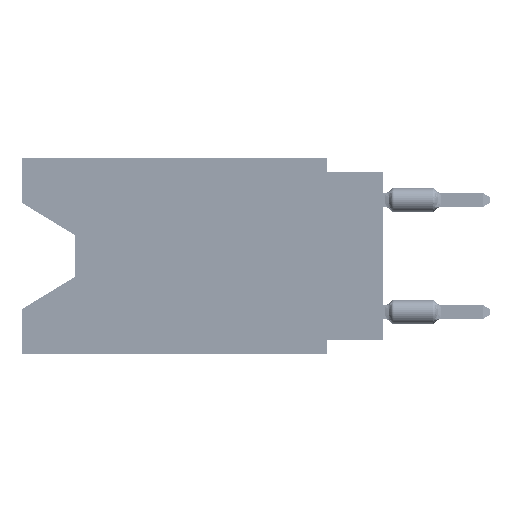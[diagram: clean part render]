
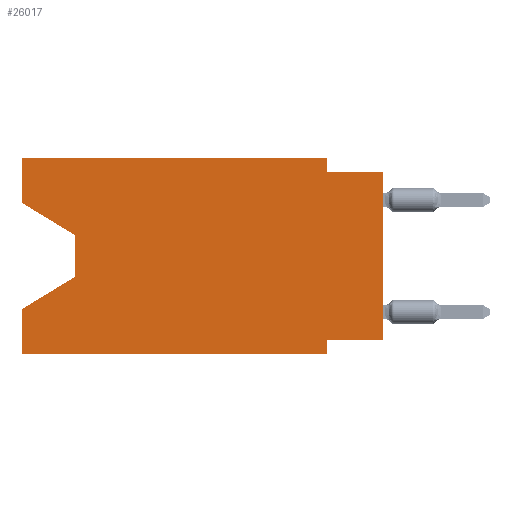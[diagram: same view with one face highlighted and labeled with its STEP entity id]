
A CAD part, left-side view. The second image highlights one B-rep face of the part: STEP entity #26017.
In plain terms, the highlighted planar face has unit normal (-1, 0, 0).
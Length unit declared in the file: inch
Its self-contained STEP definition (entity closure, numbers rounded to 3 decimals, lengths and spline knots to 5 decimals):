
#196 = DIRECTION ( 'NONE',  ( 0., 0., 1. ) ) ;
#645 = LINE ( 'NONE', #35920, #61650 ) ;
#1305 = EDGE_CURVE ( 'NONE', #66313, #22376, #6576, .T. ) ;
#3729 = FACE_OUTER_BOUND ( 'NONE', #34049, .T. ) ;
#4725 = CARTESIAN_POINT ( 'NONE',  ( 0., 0.1, -0.325 ) ) ;
#5336 = VECTOR ( 'NONE', #64543, 39.37008 ) ;
#5364 = VECTOR ( 'NONE', #60416, 39.37008 ) ;
#6576 = LINE ( 'NONE', #7235, #58800 ) ;
#7235 = CARTESIAN_POINT ( 'NONE',  ( 0., 0., 0. ) ) ;
#7884 = VECTOR ( 'NONE', #54896, 39.37008 ) ;
#8128 = LINE ( 'NONE', #8451, #54792 ) ;
#8451 = CARTESIAN_POINT ( 'NONE',  ( 0., 0.1, 0. ) ) ;
#8800 = VERTEX_POINT ( 'NONE', #4725 ) ;
#9898 = CARTESIAN_POINT ( 'NONE',  ( 0., 0.1, -0.025 ) ) ;
#12039 = CARTESIAN_POINT ( 'NONE',  ( 0., 0.55, -0.212 ) ) ;
#14314 = ORIENTED_EDGE ( 'NONE', *, *, #38287, .T. ) ;
#14531 = VERTEX_POINT ( 'NONE', #9898 ) ;
#15044 = LINE ( 'NONE', #24134, #5364 ) ;
#15332 = ORIENTED_EDGE ( 'NONE', *, *, #54161, .F. ) ;
#15468 = DIRECTION ( 'NONE',  ( 0., -1., 0. ) ) ;
#16245 = CARTESIAN_POINT ( 'NONE',  ( 0., 0., -0.325 ) ) ;
#17329 = DIRECTION ( 'NONE',  ( 0., 0., 1. ) ) ;
#17467 = VERTEX_POINT ( 'NONE', #55466 ) ;
#17940 = EDGE_CURVE ( 'NONE', #18446, #19204, #31097, .T. ) ;
#18165 = VECTOR ( 'NONE', #15468, 39.37008 ) ;
#18313 = ORIENTED_EDGE ( 'NONE', *, *, #61068, .F. ) ;
#18446 = VERTEX_POINT ( 'NONE', #41089 ) ;
#19191 = CARTESIAN_POINT ( 'NONE',  ( 0., 0.55, -0.138 ) ) ;
#19204 = VERTEX_POINT ( 'NONE', #29664 ) ;
#19906 = ORIENTED_EDGE ( 'NONE', *, *, #1305, .T. ) ;
#19976 = EDGE_CURVE ( 'NONE', #8800, #17467, #20019, .T. ) ;
#20019 = LINE ( 'NONE', #45213, #60106 ) ;
#22151 = CARTESIAN_POINT ( 'NONE',  ( 0., 0.645, -0.35 ) ) ;
#22376 = VERTEX_POINT ( 'NONE', #64152 ) ;
#23196 = LINE ( 'NONE', #49394, #53445 ) ;
#24099 = VECTOR ( 'NONE', #51792, 39.37008 ) ;
#24134 = CARTESIAN_POINT ( 'NONE',  ( 0., 0.645, 0. ) ) ;
#24540 = CARTESIAN_POINT ( 'NONE',  ( 0., 0.645, 0. ) ) ;
#24796 = ORIENTED_EDGE ( 'NONE', *, *, #57438, .T. ) ;
#24832 = VECTOR ( 'NONE', #51161, 39.37008 ) ;
#26017 = ADVANCED_FACE ( 'NONE', ( #3729 ), #44042, .F. ) ;
#27193 = AXIS2_PLACEMENT_3D ( 'NONE', #24540, #33620, #39984 ) ;
#27282 = VERTEX_POINT ( 'NONE', #32288 ) ;
#27933 = CARTESIAN_POINT ( 'NONE',  ( 0., 0.645, -0.26975 ) ) ;
#28638 = CARTESIAN_POINT ( 'NONE',  ( 0., 0.1, 0. ) ) ;
#29664 = CARTESIAN_POINT ( 'NONE',  ( 0., 0.645, 0. ) ) ;
#30184 = VERTEX_POINT ( 'NONE', #27933 ) ;
#30441 = CARTESIAN_POINT ( 'NONE',  ( 0., 0.645, 0. ) ) ;
#31097 = LINE ( 'NONE', #30441, #46076 ) ;
#31357 = VERTEX_POINT ( 'NONE', #22151 ) ;
#31621 = ORIENTED_EDGE ( 'NONE', *, *, #40860, .T. ) ;
#31747 = ORIENTED_EDGE ( 'NONE', *, *, #33072, .F. ) ;
#32288 = CARTESIAN_POINT ( 'NONE',  ( 0., 0.55, -0.138 ) ) ;
#33072 = EDGE_CURVE ( 'NONE', #14531, #22376, #40964, .T. ) ;
#33620 = DIRECTION ( 'NONE',  ( 1., 0., 0. ) ) ;
#34049 = EDGE_LOOP ( 'NONE', ( #24796, #40447, #14314, #15332, #31621, #59224, #18313, #19906, #31747, #59363, #45649, #40427 ) ) ;
#34108 = EDGE_CURVE ( 'NONE', #27282, #58447, #65201, .T. ) ;
#35920 = CARTESIAN_POINT ( 'NONE',  ( 0., 0.645, 0. ) ) ;
#38287 = EDGE_CURVE ( 'NONE', #58447, #30184, #52991, .T. ) ;
#38573 = CARTESIAN_POINT ( 'NONE',  ( 0., 0., -0.325 ) ) ;
#39984 = DIRECTION ( 'NONE',  ( 0., 0., -1. ) ) ;
#40427 = ORIENTED_EDGE ( 'NONE', *, *, #17940, .F. ) ;
#40447 = ORIENTED_EDGE ( 'NONE', *, *, #34108, .T. ) ;
#40860 = EDGE_CURVE ( 'NONE', #31357, #17467, #66246, .T. ) ;
#40964 = LINE ( 'NONE', #61475, #18165 ) ;
#41089 = CARTESIAN_POINT ( 'NONE',  ( 0., 0.645, -0.08025 ) ) ;
#43684 = DIRECTION ( 'NONE',  ( 0., -0.855, -0.519 ) ) ;
#44042 = PLANE ( 'NONE',  #27193 ) ;
#45213 = CARTESIAN_POINT ( 'NONE',  ( 0., 0.1, -0.35 ) ) ;
#45428 = CARTESIAN_POINT ( 'NONE',  ( 0., 0.645, -0.35 ) ) ;
#45569 = EDGE_CURVE ( 'NONE', #19204, #57040, #645, .T. ) ;
#45649 = ORIENTED_EDGE ( 'NONE', *, *, #45569, .F. ) ;
#46076 = VECTOR ( 'NONE', #196, 39.37008 ) ;
#49165 = CARTESIAN_POINT ( 'NONE',  ( 0., 0.55, -0.212 ) ) ;
#49394 = CARTESIAN_POINT ( 'NONE',  ( 0., 0.645, -0.08025 ) ) ;
#51161 = DIRECTION ( 'NONE',  ( 0., 1., 0. ) ) ;
#51376 = DIRECTION ( 'NONE',  ( 0., -1., 0. ) ) ;
#51792 = DIRECTION ( 'NONE',  ( 0., -1., 0. ) ) ;
#52991 = LINE ( 'NONE', #12039, #7884 ) ;
#53445 = VECTOR ( 'NONE', #43684, 39.37008 ) ;
#54161 = EDGE_CURVE ( 'NONE', #31357, #30184, #15044, .T. ) ;
#54792 = VECTOR ( 'NONE', #59192, 39.37008 ) ;
#54896 = DIRECTION ( 'NONE',  ( 0., 0.855, -0.519 ) ) ;
#55466 = CARTESIAN_POINT ( 'NONE',  ( 0., 0.1, -0.35 ) ) ;
#56284 = DIRECTION ( 'NONE',  ( 0., 0., -1. ) ) ;
#57040 = VERTEX_POINT ( 'NONE', #28638 ) ;
#57438 = EDGE_CURVE ( 'NONE', #18446, #27282, #23196, .T. ) ;
#58447 = VERTEX_POINT ( 'NONE', #49165 ) ;
#58800 = VECTOR ( 'NONE', #17329, 39.37008 ) ;
#59192 = DIRECTION ( 'NONE',  ( 0., 0., -1. ) ) ;
#59224 = ORIENTED_EDGE ( 'NONE', *, *, #19976, .F. ) ;
#59363 = ORIENTED_EDGE ( 'NONE', *, *, #60089, .F. ) ;
#60089 = EDGE_CURVE ( 'NONE', #57040, #14531, #8128, .T. ) ;
#60106 = VECTOR ( 'NONE', #56284, 39.37008 ) ;
#60416 = DIRECTION ( 'NONE',  ( 0., 0., 1. ) ) ;
#61068 = EDGE_CURVE ( 'NONE', #66313, #8800, #62261, .T. ) ;
#61475 = CARTESIAN_POINT ( 'NONE',  ( 0., 0., -0.025 ) ) ;
#61650 = VECTOR ( 'NONE', #51376, 39.37008 ) ;
#62261 = LINE ( 'NONE', #16245, #24832 ) ;
#64152 = CARTESIAN_POINT ( 'NONE',  ( 0., 0., -0.025 ) ) ;
#64543 = DIRECTION ( 'NONE',  ( 0., 0., -1. ) ) ;
#65201 = LINE ( 'NONE', #19191, #5336 ) ;
#66246 = LINE ( 'NONE', #45428, #24099 ) ;
#66313 = VERTEX_POINT ( 'NONE', #38573 ) ;
